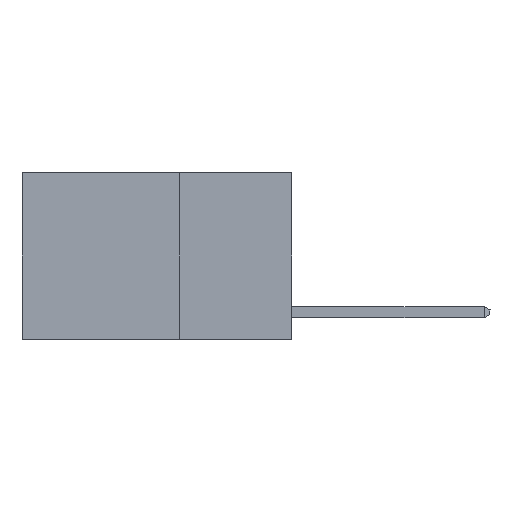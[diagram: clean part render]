
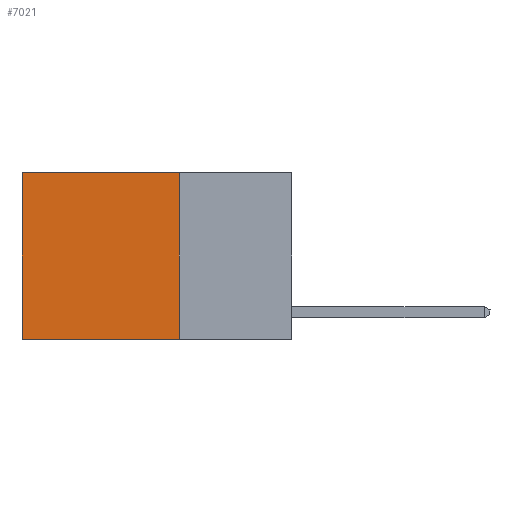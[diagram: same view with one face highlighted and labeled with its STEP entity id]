
A CAD part, left-side view. The second image highlights one B-rep face of the part: STEP entity #7021.
In plain terms, the highlighted planar face has unit normal (-1, 0, 0).
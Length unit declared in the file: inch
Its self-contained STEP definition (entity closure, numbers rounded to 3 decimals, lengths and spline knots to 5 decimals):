
#14 = CARTESIAN_POINT ( 'NONE',  ( 0.2625, 0.6, -0.37 ) ) ;
#323 = EDGE_CURVE ( 'NONE', #5550, #2219, #712, .T. ) ;
#481 = DIRECTION ( 'NONE',  ( 0., 1., 0. ) ) ;
#590 = CARTESIAN_POINT ( 'NONE',  ( 0.2625, 0.25, 0. ) ) ;
#695 = ORIENTED_EDGE ( 'NONE', *, *, #323, .T. ) ;
#712 = LINE ( 'NONE', #590, #8293 ) ;
#1346 = VERTEX_POINT ( 'NONE', #14 ) ;
#2138 = DIRECTION ( 'NONE',  ( 0., 0., -1. ) ) ;
#2219 = VERTEX_POINT ( 'NONE', #7013 ) ;
#3807 = LINE ( 'NONE', #15818, #16930 ) ;
#3949 = CARTESIAN_POINT ( 'NONE',  ( 0.2625, 0.25, 0. ) ) ;
#4795 = DIRECTION ( 'NONE',  ( 0., 0., -1. ) ) ;
#4973 = FACE_OUTER_BOUND ( 'NONE', #7361, .T. ) ;
#5094 = CARTESIAN_POINT ( 'NONE',  ( 0.2625, 0.25, -0.37 ) ) ;
#5550 = VERTEX_POINT ( 'NONE', #3949 ) ;
#6036 = ORIENTED_EDGE ( 'NONE', *, *, #8600, .F. ) ;
#6184 = EDGE_CURVE ( 'NONE', #5550, #8348, #15748, .T. ) ;
#6278 = CARTESIAN_POINT ( 'NONE',  ( 0.2625, 0.25, 0. ) ) ;
#7013 = CARTESIAN_POINT ( 'NONE',  ( 0.2625, 0.6, 0. ) ) ;
#7021 = ADVANCED_FACE ( 'NONE', ( #4973 ), #11739, .F. ) ;
#7361 = EDGE_LOOP ( 'NONE', ( #10488, #6036, #14685, #695 ) ) ;
#7680 = AXIS2_PLACEMENT_3D ( 'NONE', #6278, #15875, #2138 ) ;
#7847 = EDGE_CURVE ( 'NONE', #2219, #1346, #13741, .T. ) ;
#8293 = VECTOR ( 'NONE', #13094, 39.37008 ) ;
#8348 = VERTEX_POINT ( 'NONE', #5094 ) ;
#8493 = VECTOR ( 'NONE', #14728, 39.37008 ) ;
#8600 = EDGE_CURVE ( 'NONE', #8348, #1346, #3807, .T. ) ;
#8841 = VECTOR ( 'NONE', #4795, 39.37008 ) ;
#10488 = ORIENTED_EDGE ( 'NONE', *, *, #7847, .T. ) ;
#11655 = CARTESIAN_POINT ( 'NONE',  ( 0.2625, 0.6, 0. ) ) ;
#11739 = PLANE ( 'NONE',  #7680 ) ;
#13094 = DIRECTION ( 'NONE',  ( 0., 1., 0. ) ) ;
#13741 = LINE ( 'NONE', #11655, #8841 ) ;
#14685 = ORIENTED_EDGE ( 'NONE', *, *, #6184, .F. ) ;
#14728 = DIRECTION ( 'NONE',  ( 0., 0., -1. ) ) ;
#15748 = LINE ( 'NONE', #17436, #8493 ) ;
#15818 = CARTESIAN_POINT ( 'NONE',  ( 0.2625, 0.25, -0.37 ) ) ;
#15875 = DIRECTION ( 'NONE',  ( 1., 0., 0. ) ) ;
#16930 = VECTOR ( 'NONE', #481, 39.37008 ) ;
#17436 = CARTESIAN_POINT ( 'NONE',  ( 0.2625, 0.25, 0. ) ) ;
